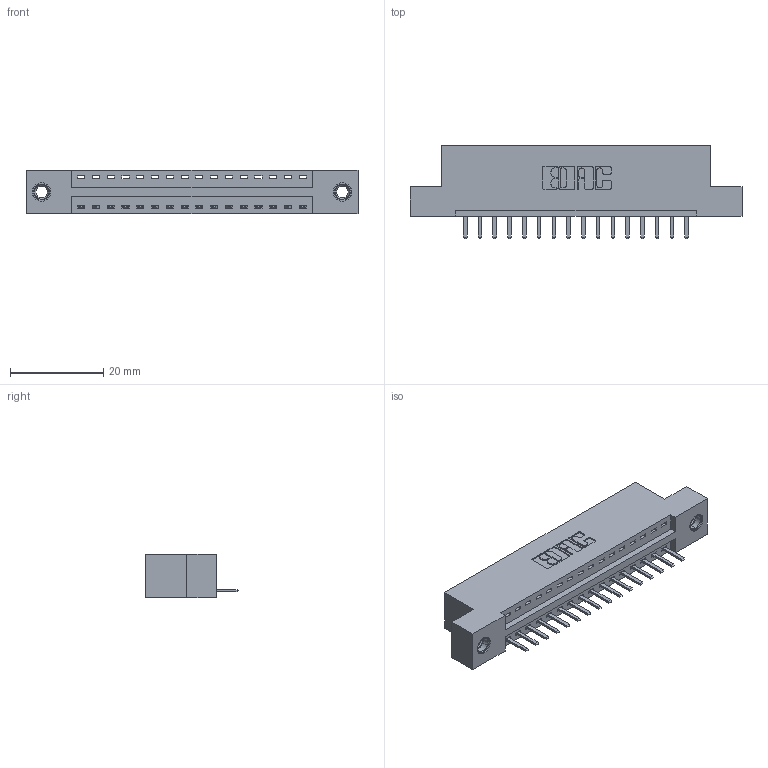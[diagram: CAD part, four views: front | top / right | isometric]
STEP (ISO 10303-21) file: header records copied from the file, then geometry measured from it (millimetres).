
FILE_DESCRIPTION (( 'STEP AP203' ), '1' );
FILE_NAME ('346-016-520-107.STEP', '2018-08-20T03:31:32', ( '' ), ( '' ), 'SwSTEP 2.0', 'SolidWorks 2016', '' );
FILE_SCHEMA (( 'CONFIG_CONTROL_DESIGN' ));
Length unit declared in the file: inch
Products named in the file (4): 346-016-520-107; 346 Part_Flush Mounting Lugs - 0.156 Dia-TI; 345-292-001_345-293-120; 345-250-001_345-250-005-103
Assembly tree (19 placements, depth 2):
  346-016-520-107
    346 Part_Flush Mounting Lugs - 0.156 Dia-TI
    345-292-001_345-293-120  x16
    345-250-001_345-250-005-103  x2
Bounding box: 71.37 x 20.02 x 9.4 mm (x, y, z)
Volume: 6593.4 mm3; surface area: 7841.3 mm2
Topology: 19 solids, 19 shells, 1174 faces, 3409 edges, 2222 vertices
Faces by surface type: plane 780, cylinder 378, cone 12, torus 4
Entity records: 14730 total; most frequent: CARTESIAN_POINT 2527, ORIENTED_EDGE 2458, DIRECTION 2275, EDGE_CURVE 1229, LINE 1009, VECTOR 1009, VERTEX_POINT 812, AXIS2_PLACEMENT_3D 633
